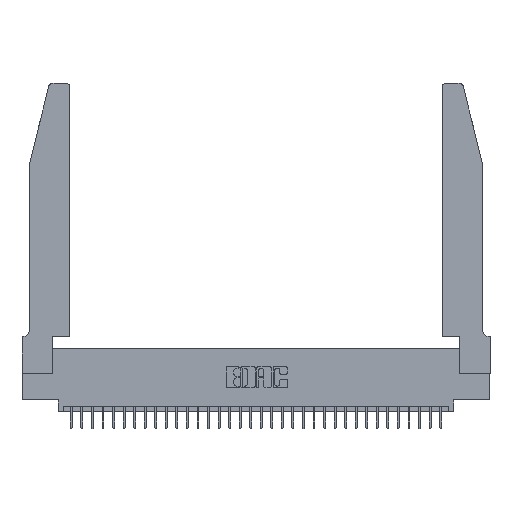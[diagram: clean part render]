
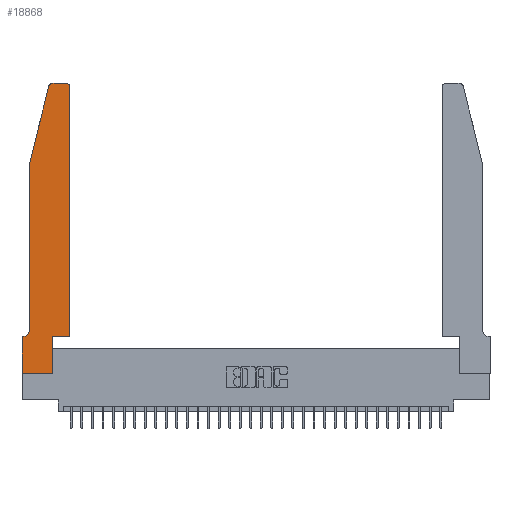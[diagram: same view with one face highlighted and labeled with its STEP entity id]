
A CAD part, top view. The second image highlights one B-rep face of the part: STEP entity #18868.
In plain terms, the highlighted planar face has unit normal (0, 0, 1).
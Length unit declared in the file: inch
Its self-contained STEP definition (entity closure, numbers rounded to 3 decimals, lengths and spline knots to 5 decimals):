
#23 = EDGE_CURVE ( 'NONE', #3123, #18370, #7585, .T. ) ;
#483 = DIRECTION ( 'NONE',  ( -0.239, -0.971, 0. ) ) ;
#622 = ORIENTED_EDGE ( 'NONE', *, *, #3282, .T. ) ;
#676 = CARTESIAN_POINT ( 'NONE',  ( 0.284, 2.72, 0.37 ) ) ;
#715 = DIRECTION ( 'NONE',  ( -1., 0., 0. ) ) ;
#757 = LINE ( 'NONE', #32779, #33280 ) ;
#1103 = CIRCLE ( 'NONE', #8230, 0.03 ) ;
#1480 = CARTESIAN_POINT ( 'NONE',  ( 0.284, 2.75, 0.37 ) ) ;
#1694 = DIRECTION ( 'NONE',  ( -1., 0., 0. ) ) ;
#1717 = CARTESIAN_POINT ( 'NONE',  ( 0.2865, 0., 0.37 ) ) ;
#1727 = DIRECTION ( 'NONE',  ( 1., 0., 0. ) ) ;
#2176 = LINE ( 'NONE', #33336, #15405 ) ;
#2529 = EDGE_CURVE ( 'NONE', #20311, #21110, #1103, .T. ) ;
#2734 = AXIS2_PLACEMENT_3D ( 'NONE', #31069, #20246, #4496 ) ;
#2854 = VERTEX_POINT ( 'NONE', #29511 ) ;
#3123 = VERTEX_POINT ( 'NONE', #23165 ) ;
#3207 = VECTOR ( 'NONE', #4530, 39.37008 ) ;
#3282 = EDGE_CURVE ( 'NONE', #7017, #2854, #15687, .T. ) ;
#3400 = EDGE_CURVE ( 'NONE', #2854, #15299, #28746, .T. ) ;
#3642 = AXIS2_PLACEMENT_3D ( 'NONE', #17209, #24832, #9276 ) ;
#4496 = DIRECTION ( 'NONE',  ( 1., 0., 0. ) ) ;
#4530 = DIRECTION ( 'NONE',  ( 0., -1., 0. ) ) ;
#4935 = EDGE_LOOP ( 'NONE', ( #24816, #18144, #27815, #10133, #622, #17363, #13662, #30898, #15158, #7150, #21916, #25122 ) ) ;
#5658 = CARTESIAN_POINT ( 'NONE',  ( 0.2865, 0.35, 0.37 ) ) ;
#6356 = PLANE ( 'NONE',  #3642 ) ;
#6390 = CARTESIAN_POINT ( 'NONE',  ( 0.25487, 2.72718, 0.37 ) ) ;
#6788 = CARTESIAN_POINT ( 'NONE',  ( 0.0755, 2., 0.37 ) ) ;
#6881 = LINE ( 'NONE', #13783, #22902 ) ;
#7017 = VERTEX_POINT ( 'NONE', #15248 ) ;
#7150 = ORIENTED_EDGE ( 'NONE', *, *, #22877, .T. ) ;
#7365 = VECTOR ( 'NONE', #29855, 39.37008 ) ;
#7585 = LINE ( 'NONE', #10632, #11729 ) ;
#7651 = DIRECTION ( 'NONE',  ( 1., 0., 0. ) ) ;
#7774 = LINE ( 'NONE', #33368, #7365 ) ;
#8200 = VERTEX_POINT ( 'NONE', #12280 ) ;
#8230 = AXIS2_PLACEMENT_3D ( 'NONE', #676, #23348, #7651 ) ;
#9145 = DIRECTION ( 'NONE',  ( 1., 0., 0. ) ) ;
#9276 = DIRECTION ( 'NONE',  ( 1., 0., 0. ) ) ;
#9326 = DIRECTION ( 'NONE',  ( 0., -1., 0. ) ) ;
#10133 = ORIENTED_EDGE ( 'NONE', *, *, #33954, .T. ) ;
#10189 = CARTESIAN_POINT ( 'NONE',  ( 0.4205, 2.75, 0.37 ) ) ;
#10632 = CARTESIAN_POINT ( 'NONE',  ( 0.4505, 0.35, 0.37 ) ) ;
#11331 = CIRCLE ( 'NONE', #2734, 0.03 ) ;
#11729 = VECTOR ( 'NONE', #28867, 39.37008 ) ;
#12280 = CARTESIAN_POINT ( 'NONE',  ( 0., 0., 0.37 ) ) ;
#12345 = LINE ( 'NONE', #12528, #3207 ) ;
#12528 = CARTESIAN_POINT ( 'NONE',  ( 0.0755, 2., 0.37 ) ) ;
#13662 = ORIENTED_EDGE ( 'NONE', *, *, #27118, .T. ) ;
#13783 = CARTESIAN_POINT ( 'NONE',  ( 0.0755, 2., 0.37 ) ) ;
#15158 = ORIENTED_EDGE ( 'NONE', *, *, #34024, .T. ) ;
#15248 = CARTESIAN_POINT ( 'NONE',  ( 0.0755, 0.42, 0.37 ) ) ;
#15299 = VERTEX_POINT ( 'NONE', #15790 ) ;
#15359 = CARTESIAN_POINT ( 'NONE',  ( 0.4505, 2.72, 0.37 ) ) ;
#15405 = VECTOR ( 'NONE', #1727, 39.37008 ) ;
#15687 = CIRCLE ( 'NONE', #33958, 0.07 ) ;
#15790 = CARTESIAN_POINT ( 'NONE',  ( 0., 0.35, 0.37 ) ) ;
#16433 = VECTOR ( 'NONE', #715, 39.37008 ) ;
#16993 = EDGE_CURVE ( 'NONE', #21110, #25322, #6881, .T. ) ;
#17209 = CARTESIAN_POINT ( 'NONE',  ( 0., 0.35, 0.37 ) ) ;
#17363 = ORIENTED_EDGE ( 'NONE', *, *, #3400, .T. ) ;
#17618 = CARTESIAN_POINT ( 'NONE',  ( 0.2605, 2.75, 0.37 ) ) ;
#18144 = ORIENTED_EDGE ( 'NONE', *, *, #2529, .T. ) ;
#18363 = EDGE_CURVE ( 'NONE', #18370, #22973, #11331, .T. ) ;
#18370 = VERTEX_POINT ( 'NONE', #15359 ) ;
#18868 = ADVANCED_FACE ( 'NONE', ( #29333 ), #6356, .T. ) ;
#20246 = DIRECTION ( 'NONE',  ( 0., 0., 1. ) ) ;
#20311 = VERTEX_POINT ( 'NONE', #1480 ) ;
#20367 = VECTOR ( 'NONE', #9326, 39.37008 ) ;
#20443 = VERTEX_POINT ( 'NONE', #1717 ) ;
#21006 = DIRECTION ( 'NONE',  ( -1., 0., 0. ) ) ;
#21110 = VERTEX_POINT ( 'NONE', #6390 ) ;
#21326 = CARTESIAN_POINT ( 'NONE',  ( 0.0055, 0.42, 0.37 ) ) ;
#21753 = CARTESIAN_POINT ( 'NONE',  ( 0.0755, 0.35, 0.37 ) ) ;
#21916 = ORIENTED_EDGE ( 'NONE', *, *, #23, .T. ) ;
#22877 = EDGE_CURVE ( 'NONE', #30885, #3123, #2176, .T. ) ;
#22902 = VECTOR ( 'NONE', #483, 39.37008 ) ;
#22973 = VERTEX_POINT ( 'NONE', #10189 ) ;
#23165 = CARTESIAN_POINT ( 'NONE',  ( 0.4505, 0.35, 0.37 ) ) ;
#23348 = DIRECTION ( 'NONE',  ( 0., 0., 1. ) ) ;
#24816 = ORIENTED_EDGE ( 'NONE', *, *, #29910, .T. ) ;
#24832 = DIRECTION ( 'NONE',  ( 0., 0., 1. ) ) ;
#24840 = LINE ( 'NONE', #32490, #20367 ) ;
#25122 = ORIENTED_EDGE ( 'NONE', *, *, #18363, .T. ) ;
#25322 = VERTEX_POINT ( 'NONE', #6788 ) ;
#26612 = DIRECTION ( 'NONE',  ( 0., 0., -1. ) ) ;
#27118 = EDGE_CURVE ( 'NONE', #15299, #8200, #24840, .T. ) ;
#27815 = ORIENTED_EDGE ( 'NONE', *, *, #16993, .T. ) ;
#28746 = LINE ( 'NONE', #21753, #16433 ) ;
#28847 = VECTOR ( 'NONE', #1694, 39.37008 ) ;
#28867 = DIRECTION ( 'NONE',  ( 0., 1., 0. ) ) ;
#29333 = FACE_OUTER_BOUND ( 'NONE', #4935, .T. ) ;
#29511 = CARTESIAN_POINT ( 'NONE',  ( 0.0055, 0.35, 0.37 ) ) ;
#29855 = DIRECTION ( 'NONE',  ( 0., 1., 0. ) ) ;
#29910 = EDGE_CURVE ( 'NONE', #22973, #20311, #32137, .T. ) ;
#30885 = VERTEX_POINT ( 'NONE', #5658 ) ;
#30898 = ORIENTED_EDGE ( 'NONE', *, *, #31092, .T. ) ;
#31069 = CARTESIAN_POINT ( 'NONE',  ( 0.4205, 2.72, 0.37 ) ) ;
#31092 = EDGE_CURVE ( 'NONE', #8200, #20443, #757, .T. ) ;
#32137 = LINE ( 'NONE', #17618, #28847 ) ;
#32490 = CARTESIAN_POINT ( 'NONE',  ( 0., 0., 0.37 ) ) ;
#32779 = CARTESIAN_POINT ( 'NONE',  ( 0., 0., 0.37 ) ) ;
#33280 = VECTOR ( 'NONE', #9145, 39.37008 ) ;
#33336 = CARTESIAN_POINT ( 'NONE',  ( 0.4505, 0.35, 0.37 ) ) ;
#33368 = CARTESIAN_POINT ( 'NONE',  ( 0.2865, 0.35, 0.37 ) ) ;
#33954 = EDGE_CURVE ( 'NONE', #25322, #7017, #12345, .T. ) ;
#33958 = AXIS2_PLACEMENT_3D ( 'NONE', #21326, #26612, #21006 ) ;
#34024 = EDGE_CURVE ( 'NONE', #20443, #30885, #7774, .T. ) ;
